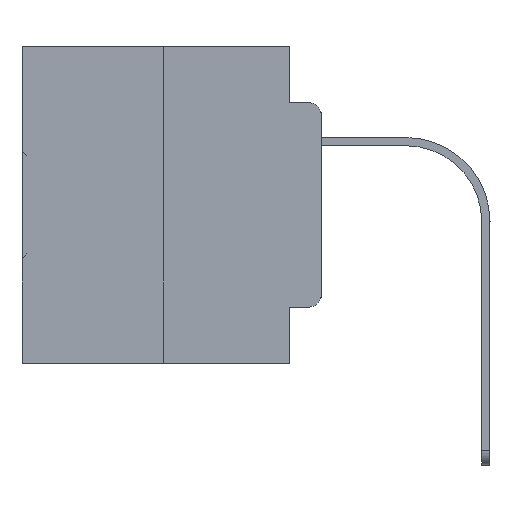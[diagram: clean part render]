
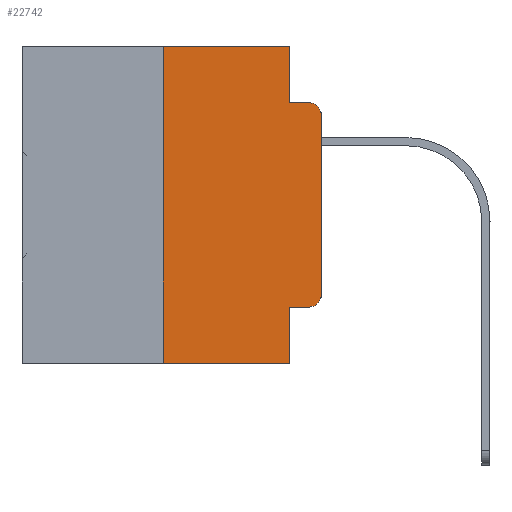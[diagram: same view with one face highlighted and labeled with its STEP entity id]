
A CAD part, left-side view. The second image highlights one B-rep face of the part: STEP entity #22742.
In plain terms, the highlighted planar face has unit normal (-1, 0, 0).
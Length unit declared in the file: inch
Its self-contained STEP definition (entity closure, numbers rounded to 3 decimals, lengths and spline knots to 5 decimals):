
#71 = VECTOR ( 'NONE', #11043, 39.37008 ) ;
#134 = DIRECTION ( 'NONE',  ( 0., 0., -1. ) ) ;
#600 = ORIENTED_EDGE ( 'NONE', *, *, #7945, .T. ) ;
#614 = LINE ( 'NONE', #28047, #31399 ) ;
#686 = ORIENTED_EDGE ( 'NONE', *, *, #31159, .F. ) ;
#704 = LINE ( 'NONE', #8386, #17442 ) ;
#1216 = EDGE_CURVE ( 'NONE', #14036, #23218, #22120, .T. ) ;
#1759 = LINE ( 'NONE', #29498, #13835 ) ;
#1935 = VERTEX_POINT ( 'NONE', #9494 ) ;
#1996 = ORIENTED_EDGE ( 'NONE', *, *, #12673, .F. ) ;
#3491 = DIRECTION ( 'NONE',  ( 0., 0., -1. ) ) ;
#3912 = PLANE ( 'NONE',  #28876 ) ;
#4186 = ORIENTED_EDGE ( 'NONE', *, *, #20906, .F. ) ;
#4870 = DIRECTION ( 'NONE',  ( 0., 0., 1. ) ) ;
#4990 = CARTESIAN_POINT ( 'NONE',  ( 0., 0.02, -0.1085 ) ) ;
#6464 = ORIENTED_EDGE ( 'NONE', *, *, #30843, .T. ) ;
#6796 = AXIS2_PLACEMENT_3D ( 'NONE', #4990, #27974, #3491 ) ;
#7945 = EDGE_CURVE ( 'NONE', #15148, #9727, #15183, .T. ) ;
#8238 = VERTEX_POINT ( 'NONE', #22188 ) ;
#8386 = CARTESIAN_POINT ( 'NONE',  ( 0., 0.473, -0.5 ) ) ;
#8454 = CARTESIAN_POINT ( 'NONE',  ( 0., 0.051, -0.4115 ) ) ;
#8795 = EDGE_LOOP ( 'NONE', ( #27625, #600, #22097, #4186, #686, #31612, #19595, #1996, #6464, #28618 ) ) ;
#9494 = CARTESIAN_POINT ( 'NONE',  ( 0., 0.051, -0.0885 ) ) ;
#9727 = VERTEX_POINT ( 'NONE', #26103 ) ;
#10617 = EDGE_CURVE ( 'NONE', #8238, #19197, #704, .T. ) ;
#10864 = DIRECTION ( 'NONE',  ( 0., -1., 0. ) ) ;
#11043 = DIRECTION ( 'NONE',  ( 0., -1., 0. ) ) ;
#12208 = CARTESIAN_POINT ( 'NONE',  ( 0., 0., -0.3915 ) ) ;
#12673 = EDGE_CURVE ( 'NONE', #23164, #19197, #1759, .T. ) ;
#13218 = VECTOR ( 'NONE', #32417, 39.37008 ) ;
#13835 = VECTOR ( 'NONE', #24423, 39.37008 ) ;
#14017 = EDGE_CURVE ( 'NONE', #23218, #15148, #25059, .T. ) ;
#14036 = VERTEX_POINT ( 'NONE', #25395 ) ;
#14201 = VERTEX_POINT ( 'NONE', #26186 ) ;
#15148 = VERTEX_POINT ( 'NONE', #15889 ) ;
#15183 = CIRCLE ( 'NONE', #6796, 0.02 ) ;
#15710 = CARTESIAN_POINT ( 'NONE',  ( 0., 0.051, -0.4115 ) ) ;
#15889 = CARTESIAN_POINT ( 'NONE',  ( 0., 0., -0.1085 ) ) ;
#15995 = CARTESIAN_POINT ( 'NONE',  ( 0., 0.051, -0.0885 ) ) ;
#16919 = LINE ( 'NONE', #15995, #71 ) ;
#17442 = VECTOR ( 'NONE', #10864, 39.37008 ) ;
#17533 = DIRECTION ( 'NONE',  ( 0., 0., 1. ) ) ;
#18191 = LINE ( 'NONE', #15710, #32084 ) ;
#18703 = FACE_OUTER_BOUND ( 'NONE', #8795, .T. ) ;
#19197 = VERTEX_POINT ( 'NONE', #30204 ) ;
#19493 = DIRECTION ( 'NONE',  ( 0., 0., -1. ) ) ;
#19506 = AXIS2_PLACEMENT_3D ( 'NONE', #21798, #27036, #19493 ) ;
#19595 = ORIENTED_EDGE ( 'NONE', *, *, #10617, .T. ) ;
#19800 = CARTESIAN_POINT ( 'NONE',  ( 0., 0.473, 0. ) ) ;
#20836 = EDGE_CURVE ( 'NONE', #8238, #14201, #32299, .T. ) ;
#20906 = EDGE_CURVE ( 'NONE', #21294, #1935, #614, .T. ) ;
#21294 = VERTEX_POINT ( 'NONE', #32420 ) ;
#21798 = CARTESIAN_POINT ( 'NONE',  ( 0., 0.02, -0.3915 ) ) ;
#22097 = ORIENTED_EDGE ( 'NONE', *, *, #23495, .F. ) ;
#22120 = CIRCLE ( 'NONE', #19506, 0.02 ) ;
#22188 = CARTESIAN_POINT ( 'NONE',  ( 0., 0.25, -0.5 ) ) ;
#22742 = ADVANCED_FACE ( 'NONE', ( #18703 ), #3912, .F. ) ;
#23164 = VERTEX_POINT ( 'NONE', #8454 ) ;
#23211 = VECTOR ( 'NONE', #4870, 39.37008 ) ;
#23218 = VERTEX_POINT ( 'NONE', #12208 ) ;
#23495 = EDGE_CURVE ( 'NONE', #1935, #9727, #16919, .T. ) ;
#23953 = DIRECTION ( 'NONE',  ( 0., 0., -1. ) ) ;
#24064 = VECTOR ( 'NONE', #17533, 39.37008 ) ;
#24423 = DIRECTION ( 'NONE',  ( 0., 0., -1. ) ) ;
#25059 = LINE ( 'NONE', #25223, #23211 ) ;
#25223 = CARTESIAN_POINT ( 'NONE',  ( 0., 0., 0. ) ) ;
#25395 = CARTESIAN_POINT ( 'NONE',  ( 0., 0.02, -0.4115 ) ) ;
#25718 = DIRECTION ( 'NONE',  ( 0., -1., 0. ) ) ;
#26103 = CARTESIAN_POINT ( 'NONE',  ( 0., 0.02, -0.0885 ) ) ;
#26186 = CARTESIAN_POINT ( 'NONE',  ( 0., 0.25, 0. ) ) ;
#26557 = CARTESIAN_POINT ( 'NONE',  ( 0., 0.473, 0. ) ) ;
#27036 = DIRECTION ( 'NONE',  ( -1., 0., 0. ) ) ;
#27548 = CARTESIAN_POINT ( 'NONE',  ( 0., 0.25, 0. ) ) ;
#27625 = ORIENTED_EDGE ( 'NONE', *, *, #14017, .T. ) ;
#27974 = DIRECTION ( 'NONE',  ( -1., 0., 0. ) ) ;
#28047 = CARTESIAN_POINT ( 'NONE',  ( 0., 0.051, 0. ) ) ;
#28618 = ORIENTED_EDGE ( 'NONE', *, *, #1216, .T. ) ;
#28709 = DIRECTION ( 'NONE',  ( 1., 0., 0. ) ) ;
#28876 = AXIS2_PLACEMENT_3D ( 'NONE', #26557, #28709, #23953 ) ;
#29498 = CARTESIAN_POINT ( 'NONE',  ( 0., 0.051, 0. ) ) ;
#30204 = CARTESIAN_POINT ( 'NONE',  ( 0., 0.051, -0.5 ) ) ;
#30284 = LINE ( 'NONE', #19800, #13218 ) ;
#30843 = EDGE_CURVE ( 'NONE', #23164, #14036, #18191, .T. ) ;
#31159 = EDGE_CURVE ( 'NONE', #14201, #21294, #30284, .T. ) ;
#31399 = VECTOR ( 'NONE', #134, 39.37008 ) ;
#31612 = ORIENTED_EDGE ( 'NONE', *, *, #20836, .F. ) ;
#32084 = VECTOR ( 'NONE', #25718, 39.37008 ) ;
#32299 = LINE ( 'NONE', #27548, #24064 ) ;
#32417 = DIRECTION ( 'NONE',  ( 0., -1., 0. ) ) ;
#32420 = CARTESIAN_POINT ( 'NONE',  ( 0., 0.051, 0. ) ) ;
